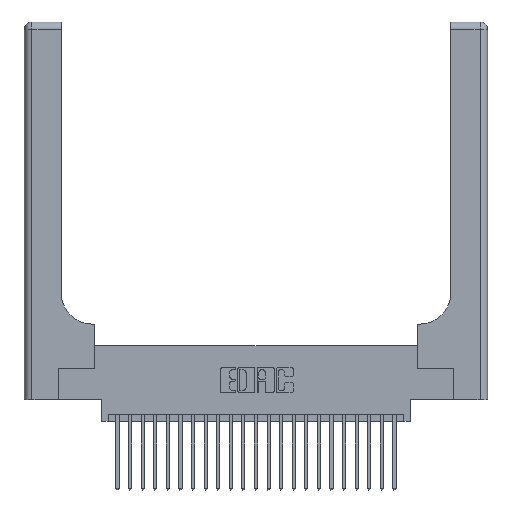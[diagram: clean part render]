
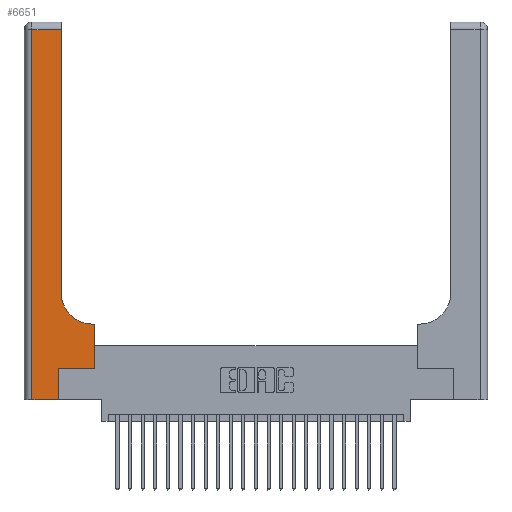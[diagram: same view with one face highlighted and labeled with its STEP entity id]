
A CAD part, top view. The second image highlights one B-rep face of the part: STEP entity #6651.
In plain terms, the highlighted planar face has unit normal (0, 0, 1).
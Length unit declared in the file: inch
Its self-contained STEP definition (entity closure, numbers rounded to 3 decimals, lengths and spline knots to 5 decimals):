
#275 = CARTESIAN_POINT ( 'NONE',  ( 0.5415, 0.6, 0.37 ) ) ;
#374 = CARTESIAN_POINT ( 'NONE',  ( 0., 0., 0.37 ) ) ;
#1100 = CARTESIAN_POINT ( 'NONE',  ( 0.5585, 0.25, 0.37 ) ) ;
#1252 = ORIENTED_EDGE ( 'NONE', *, *, #9511, .T. ) ;
#1342 = LINE ( 'NONE', #5449, #6121 ) ;
#1588 = CARTESIAN_POINT ( 'NONE',  ( 0.06, 2.94, 0.37 ) ) ;
#1796 = LINE ( 'NONE', #23632, #11928 ) ;
#1930 = CARTESIAN_POINT ( 'NONE',  ( 0.269, 0., 0.37 ) ) ;
#2068 = VERTEX_POINT ( 'NONE', #275 ) ;
#2230 = VERTEX_POINT ( 'NONE', #4782 ) ;
#2429 = DIRECTION ( 'NONE',  ( 1., 0., 0. ) ) ;
#2892 = VECTOR ( 'NONE', #9885, 39.37008 ) ;
#2983 = ORIENTED_EDGE ( 'NONE', *, *, #16725, .T. ) ;
#3387 = EDGE_CURVE ( 'NONE', #18138, #21720, #4672, .T. ) ;
#3890 = EDGE_LOOP ( 'NONE', ( #17405, #2983, #24119, #6868, #15862, #17728, #9510, #7909, #1252 ) ) ;
#4064 = VECTOR ( 'NONE', #2429, 39.37008 ) ;
#4119 = VECTOR ( 'NONE', #18007, 39.37008 ) ;
#4167 = VERTEX_POINT ( 'NONE', #13315 ) ;
#4553 = VERTEX_POINT ( 'NONE', #22700 ) ;
#4672 = LINE ( 'NONE', #374, #4064 ) ;
#4782 = CARTESIAN_POINT ( 'NONE',  ( 0.269, 0.25, 0.37 ) ) ;
#5223 = EDGE_CURVE ( 'NONE', #21720, #2230, #9541, .T. ) ;
#5449 = CARTESIAN_POINT ( 'NONE',  ( 0.2915, 0.6, 0.37 ) ) ;
#5938 = LINE ( 'NONE', #23801, #15967 ) ;
#6121 = VECTOR ( 'NONE', #9573, 39.37008 ) ;
#6563 = CARTESIAN_POINT ( 'NONE',  ( 0.5415, 0.85, 0.37 ) ) ;
#6651 = ADVANCED_FACE ( 'NONE', ( #23442 ), #16782, .F. ) ;
#6837 = DIRECTION ( 'NONE',  ( 0., 0., -1. ) ) ;
#6868 = ORIENTED_EDGE ( 'NONE', *, *, #3387, .T. ) ;
#7346 = AXIS2_PLACEMENT_3D ( 'NONE', #18770, #6837, #20811 ) ;
#7909 = ORIENTED_EDGE ( 'NONE', *, *, #22694, .T. ) ;
#8630 = DIRECTION ( 'NONE',  ( 1., 0., 0. ) ) ;
#9109 = AXIS2_PLACEMENT_3D ( 'NONE', #6563, #20544, #8630 ) ;
#9309 = DIRECTION ( 'NONE',  ( 0., -1., 0. ) ) ;
#9510 = ORIENTED_EDGE ( 'NONE', *, *, #13438, .T. ) ;
#9511 = EDGE_CURVE ( 'NONE', #2068, #16738, #9679, .T. ) ;
#9541 = LINE ( 'NONE', #1930, #4119 ) ;
#9573 = DIRECTION ( 'NONE',  ( -1., 0., 0. ) ) ;
#9679 = CIRCLE ( 'NONE', #9109, 0.25 ) ;
#9885 = DIRECTION ( 'NONE',  ( 0., 1., 0. ) ) ;
#11124 = CARTESIAN_POINT ( 'NONE',  ( 0.269, 0.25, 0.37 ) ) ;
#11928 = VECTOR ( 'NONE', #21550, 39.37008 ) ;
#12715 = VECTOR ( 'NONE', #9309, 39.37008 ) ;
#13089 = DIRECTION ( 'NONE',  ( 1., 0., 0. ) ) ;
#13315 = CARTESIAN_POINT ( 'NONE',  ( 0.2915, 2.94, 0.37 ) ) ;
#13362 = VECTOR ( 'NONE', #13089, 39.37008 ) ;
#13438 = EDGE_CURVE ( 'NONE', #24362, #4553, #18861, .T. ) ;
#13799 = CARTESIAN_POINT ( 'NONE',  ( 0.269, 0., 0.37 ) ) ;
#13974 = LINE ( 'NONE', #11124, #13362 ) ;
#15862 = ORIENTED_EDGE ( 'NONE', *, *, #5223, .T. ) ;
#15967 = VECTOR ( 'NONE', #25782, 39.37008 ) ;
#16393 = VERTEX_POINT ( 'NONE', #1588 ) ;
#16660 = EDGE_CURVE ( 'NONE', #16738, #4167, #1796, .T. ) ;
#16725 = EDGE_CURVE ( 'NONE', #4167, #16393, #5938, .T. ) ;
#16738 = VERTEX_POINT ( 'NONE', #23880 ) ;
#16782 = PLANE ( 'NONE',  #7346 ) ;
#17405 = ORIENTED_EDGE ( 'NONE', *, *, #16660, .T. ) ;
#17728 = ORIENTED_EDGE ( 'NONE', *, *, #22145, .T. ) ;
#17853 = CARTESIAN_POINT ( 'NONE',  ( 0.5585, 0.25, 0.37 ) ) ;
#18007 = DIRECTION ( 'NONE',  ( 0., 1., 0. ) ) ;
#18138 = VERTEX_POINT ( 'NONE', #22781 ) ;
#18770 = CARTESIAN_POINT ( 'NONE',  ( 0., 3., 0.37 ) ) ;
#18861 = LINE ( 'NONE', #17853, #2892 ) ;
#20544 = DIRECTION ( 'NONE',  ( 0., 0., -1. ) ) ;
#20811 = DIRECTION ( 'NONE',  ( -1., 0., 0. ) ) ;
#21550 = DIRECTION ( 'NONE',  ( 0., 1., 0. ) ) ;
#21720 = VERTEX_POINT ( 'NONE', #13799 ) ;
#22145 = EDGE_CURVE ( 'NONE', #2230, #24362, #13974, .T. ) ;
#22630 = EDGE_CURVE ( 'NONE', #16393, #18138, #23315, .T. ) ;
#22694 = EDGE_CURVE ( 'NONE', #4553, #2068, #1342, .T. ) ;
#22700 = CARTESIAN_POINT ( 'NONE',  ( 0.5585, 0.6, 0.37 ) ) ;
#22781 = CARTESIAN_POINT ( 'NONE',  ( 0.06, 0., 0.37 ) ) ;
#23221 = CARTESIAN_POINT ( 'NONE',  ( 0.06, 3., 0.37 ) ) ;
#23315 = LINE ( 'NONE', #23221, #12715 ) ;
#23442 = FACE_OUTER_BOUND ( 'NONE', #3890, .T. ) ;
#23632 = CARTESIAN_POINT ( 'NONE',  ( 0.2915, 3., 0.37 ) ) ;
#23801 = CARTESIAN_POINT ( 'NONE',  ( 0., 2.94, 0.37 ) ) ;
#23880 = CARTESIAN_POINT ( 'NONE',  ( 0.2915, 0.85, 0.37 ) ) ;
#24119 = ORIENTED_EDGE ( 'NONE', *, *, #22630, .T. ) ;
#24362 = VERTEX_POINT ( 'NONE', #1100 ) ;
#25782 = DIRECTION ( 'NONE',  ( -1., 0., 0. ) ) ;
